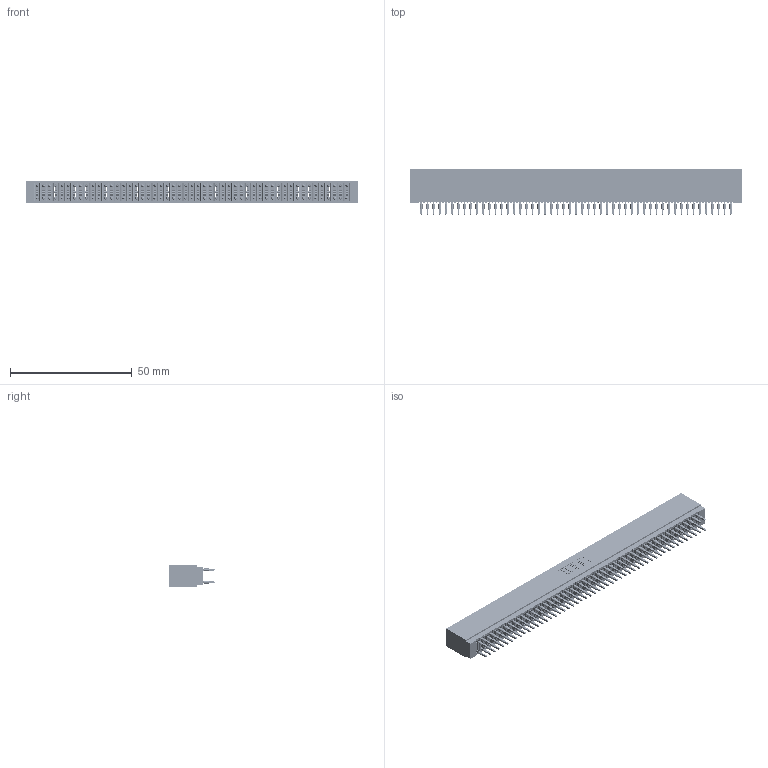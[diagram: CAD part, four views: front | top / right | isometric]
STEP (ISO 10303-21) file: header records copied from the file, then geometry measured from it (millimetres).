
FILE_DESCRIPTION (( 'STEP AP203' ), '1' );
FILE_NAME ('725-102-560-201.STEP', '2026-02-24T20:06:43', ( '' ), ( '' ), 'SwSTEP 2.0', 'SolidWorks 2023', '' );
FILE_SCHEMA (( 'CONFIG_CONTROL_DESIGN' ));
Length unit declared in the file: millimetre
Products named in the file (3): 725-102-560-201; 745-292-001_560; 725 Part_Insulator Option - 01
Assembly tree (103 placements, depth 2):
  725-102-560-201
    725 Part_Insulator Option - 01
    745-292-001_560  x102
Bounding box: 136.14 x 18.8 x 8.89 mm (x, y, z)
Volume: 11127.8 mm3; surface area: 25304.1 mm2
Topology: 103 solids, 103 shells, 10142 faces, 27743 edges, 17610 vertices
Faces by surface type: plane 5257, cylinder 2233, bspline 2040, torus 612
Entity records: 84918 total; most frequent: CARTESIAN_POINT 15229, ORIENTED_EDGE 14682, DIRECTION 12825, EDGE_CURVE 7341, LINE 6845, VECTOR 6845, VERTEX_POINT 4682, AXIS2_PLACEMENT_3D 2990
